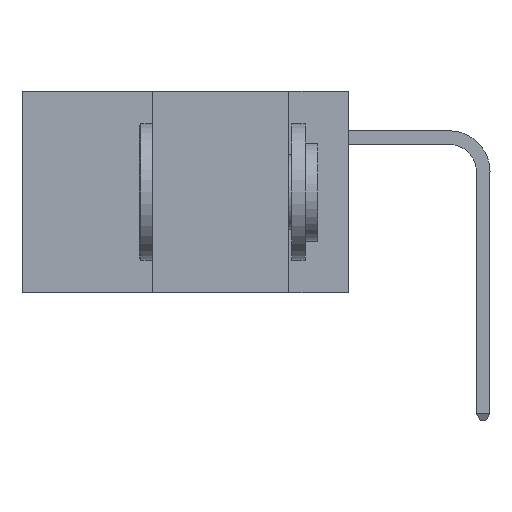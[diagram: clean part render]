
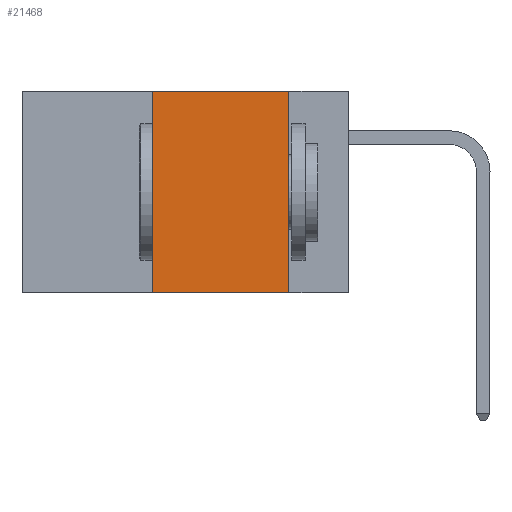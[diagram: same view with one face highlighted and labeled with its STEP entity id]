
A CAD part, left-side view. The second image highlights one B-rep face of the part: STEP entity #21468.
In plain terms, the highlighted planar face has unit normal (-1, 0, 0).
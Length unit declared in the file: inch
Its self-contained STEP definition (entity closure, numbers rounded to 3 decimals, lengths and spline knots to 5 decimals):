
#690 = CARTESIAN_POINT ( 'NONE',  ( 0., 0.6, -0.37 ) ) ;
#764 = DIRECTION ( 'NONE',  ( 0., -1., 0. ) ) ;
#1335 = AXIS2_PLACEMENT_3D ( 'NONE', #9392, #21673, #11322 ) ;
#1688 = VERTEX_POINT ( 'NONE', #3123 ) ;
#2483 = EDGE_CURVE ( 'NONE', #4705, #11706, #12109, .T. ) ;
#2830 = ORIENTED_EDGE ( 'NONE', *, *, #15542, .F. ) ;
#3123 = CARTESIAN_POINT ( 'NONE',  ( 0., 0.36, 0. ) ) ;
#3298 = EDGE_LOOP ( 'NONE', ( #12940, #12429, #2830, #8286 ) ) ;
#4077 = DIRECTION ( 'NONE',  ( 0., 0., -1. ) ) ;
#4705 = VERTEX_POINT ( 'NONE', #15031 ) ;
#4757 = VECTOR ( 'NONE', #8655, 39.37008 ) ;
#4837 = VERTEX_POINT ( 'NONE', #21413 ) ;
#7794 = DIRECTION ( 'NONE',  ( 0., 0., 1. ) ) ;
#8154 = VECTOR ( 'NONE', #7794, 39.37008 ) ;
#8286 = ORIENTED_EDGE ( 'NONE', *, *, #14101, .T. ) ;
#8619 = VECTOR ( 'NONE', #764, 39.37008 ) ;
#8655 = DIRECTION ( 'NONE',  ( 0., -1., 0. ) ) ;
#9392 = CARTESIAN_POINT ( 'NONE',  ( 0., 0.6, 0. ) ) ;
#11322 = DIRECTION ( 'NONE',  ( 0., 0., -1. ) ) ;
#11706 = VERTEX_POINT ( 'NONE', #16871 ) ;
#12109 = LINE ( 'NONE', #12764, #17534 ) ;
#12157 = LINE ( 'NONE', #19081, #4757 ) ;
#12429 = ORIENTED_EDGE ( 'NONE', *, *, #18146, .F. ) ;
#12764 = CARTESIAN_POINT ( 'NONE',  ( 0., 0.11, 0. ) ) ;
#12940 = ORIENTED_EDGE ( 'NONE', *, *, #2483, .F. ) ;
#14101 = EDGE_CURVE ( 'NONE', #4837, #11706, #17132, .T. ) ;
#14135 = FACE_OUTER_BOUND ( 'NONE', #3298, .T. ) ;
#14736 = LINE ( 'NONE', #21750, #8154 ) ;
#15031 = CARTESIAN_POINT ( 'NONE',  ( 0., 0.11, 0. ) ) ;
#15542 = EDGE_CURVE ( 'NONE', #4837, #1688, #14736, .T. ) ;
#16532 = PLANE ( 'NONE',  #1335 ) ;
#16871 = CARTESIAN_POINT ( 'NONE',  ( 0., 0.11, -0.37 ) ) ;
#17132 = LINE ( 'NONE', #690, #8619 ) ;
#17534 = VECTOR ( 'NONE', #4077, 39.37008 ) ;
#18146 = EDGE_CURVE ( 'NONE', #1688, #4705, #12157, .T. ) ;
#19081 = CARTESIAN_POINT ( 'NONE',  ( 0., 0.6, 0. ) ) ;
#21413 = CARTESIAN_POINT ( 'NONE',  ( 0., 0.36, -0.37 ) ) ;
#21468 = ADVANCED_FACE ( 'NONE', ( #14135 ), #16532, .F. ) ;
#21673 = DIRECTION ( 'NONE',  ( 1., 0., 0. ) ) ;
#21750 = CARTESIAN_POINT ( 'NONE',  ( 0., 0.36, 0. ) ) ;
